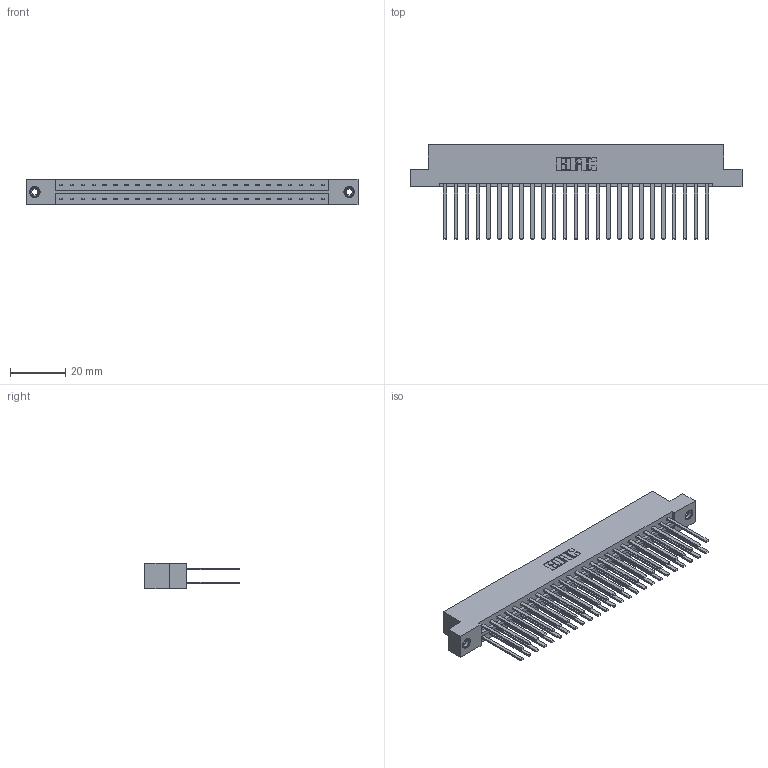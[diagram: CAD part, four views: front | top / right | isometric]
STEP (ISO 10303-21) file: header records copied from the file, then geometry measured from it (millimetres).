
FILE_DESCRIPTION (( 'STEP AP203' ), '1' );
FILE_NAME ('333-050-544-208.STEP', '2018-08-04T01:08:52', ( '' ), ( '' ), 'SwSTEP 2.0', 'SolidWorks 2016', '' );
FILE_SCHEMA (( 'CONFIG_CONTROL_DESIGN' ));
Length unit declared in the file: inch
Products named in the file (4): 333 Part_Flush - .156 Dia - TI; 345-292-001_345-293-144; 345-250-001_345-250-003-102; 333-050-544-208
Assembly tree (53 placements, depth 2):
  333-050-544-208
    333 Part_Flush - .156 Dia - TI
    345-292-001_345-293-144  x50
    345-250-001_345-250-003-102  x2
Bounding box: 120.6 x 34.3 x 9.4 mm (x, y, z)
Volume: 12847.9 mm3; surface area: 17285.2 mm2
Topology: 53 solids, 53 shells, 2474 faces, 7297 edges, 4790 vertices
Faces by surface type: plane 1702, cylinder 756, cone 12, torus 4
Entity records: 19284 total; most frequent: CARTESIAN_POINT 3197, ORIENTED_EDGE 3126, DIRECTION 2789, EDGE_CURVE 1563, LINE 1419, VECTOR 1419, VERTEX_POINT 1036, AXIS2_PLACEMENT_3D 685
